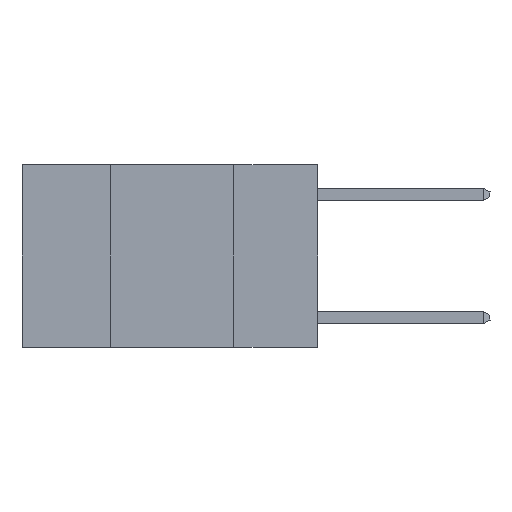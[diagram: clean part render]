
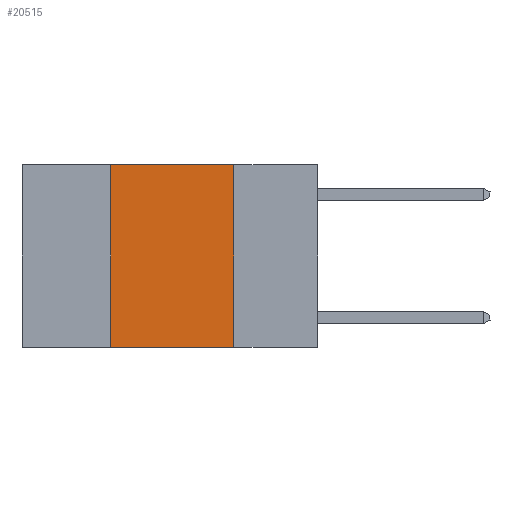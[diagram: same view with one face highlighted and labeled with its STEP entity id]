
A CAD part, left-side view. The second image highlights one B-rep face of the part: STEP entity #20515.
In plain terms, the highlighted planar face has unit normal (-1, 0, 0).
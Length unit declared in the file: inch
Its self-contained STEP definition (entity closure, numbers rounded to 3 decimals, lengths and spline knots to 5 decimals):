
#2632 = DIRECTION ( 'NONE',  ( 0., -1., 0. ) ) ;
#4172 = CARTESIAN_POINT ( 'NONE',  ( 0., 0.42, -0.37 ) ) ;
#4291 = DIRECTION ( 'NONE',  ( 0., 0., -1. ) ) ;
#4312 = PLANE ( 'NONE',  #13326 ) ;
#4443 = CARTESIAN_POINT ( 'NONE',  ( 0., 0.6, 0. ) ) ;
#4480 = EDGE_CURVE ( 'NONE', #9064, #8249, #22504, .T. ) ;
#4532 = VERTEX_POINT ( 'NONE', #4172 ) ;
#5035 = VECTOR ( 'NONE', #4291, 39.37008 ) ;
#6691 = VECTOR ( 'NONE', #2632, 39.37008 ) ;
#7535 = ORIENTED_EDGE ( 'NONE', *, *, #9464, .F. ) ;
#8249 = VERTEX_POINT ( 'NONE', #21044 ) ;
#8266 = LINE ( 'NONE', #15604, #21627 ) ;
#8502 = DIRECTION ( 'NONE',  ( 0., -1., 0. ) ) ;
#9064 = VERTEX_POINT ( 'NONE', #16887 ) ;
#9464 = EDGE_CURVE ( 'NONE', #10847, #9064, #11238, .T. ) ;
#9883 = DIRECTION ( 'NONE',  ( 1., 0., 0. ) ) ;
#10847 = VERTEX_POINT ( 'NONE', #14743 ) ;
#11238 = LINE ( 'NONE', #4443, #6691 ) ;
#11672 = CARTESIAN_POINT ( 'NONE',  ( 0., 0.6, 0. ) ) ;
#12285 = LINE ( 'NONE', #12526, #16124 ) ;
#12526 = CARTESIAN_POINT ( 'NONE',  ( 0., 0.42, 0. ) ) ;
#12556 = EDGE_CURVE ( 'NONE', #4532, #10847, #12285, .T. ) ;
#13326 = AXIS2_PLACEMENT_3D ( 'NONE', #11672, #9883, #15403 ) ;
#13495 = FACE_OUTER_BOUND ( 'NONE', #21752, .T. ) ;
#14743 = CARTESIAN_POINT ( 'NONE',  ( 0., 0.42, 0. ) ) ;
#15144 = CARTESIAN_POINT ( 'NONE',  ( 0., 0.17, 0. ) ) ;
#15403 = DIRECTION ( 'NONE',  ( 0., 0., -1. ) ) ;
#15604 = CARTESIAN_POINT ( 'NONE',  ( 0., 0.6, -0.37 ) ) ;
#16124 = VECTOR ( 'NONE', #16125, 39.37008 ) ;
#16125 = DIRECTION ( 'NONE',  ( 0., 0., 1. ) ) ;
#16887 = CARTESIAN_POINT ( 'NONE',  ( 0., 0.17, 0. ) ) ;
#18661 = ORIENTED_EDGE ( 'NONE', *, *, #19726, .T. ) ;
#19573 = ORIENTED_EDGE ( 'NONE', *, *, #4480, .F. ) ;
#19726 = EDGE_CURVE ( 'NONE', #4532, #8249, #8266, .T. ) ;
#20515 = ADVANCED_FACE ( 'NONE', ( #13495 ), #4312, .F. ) ;
#21044 = CARTESIAN_POINT ( 'NONE',  ( 0., 0.17, -0.37 ) ) ;
#21627 = VECTOR ( 'NONE', #8502, 39.37008 ) ;
#21752 = EDGE_LOOP ( 'NONE', ( #19573, #7535, #22787, #18661 ) ) ;
#22504 = LINE ( 'NONE', #15144, #5035 ) ;
#22787 = ORIENTED_EDGE ( 'NONE', *, *, #12556, .F. ) ;
